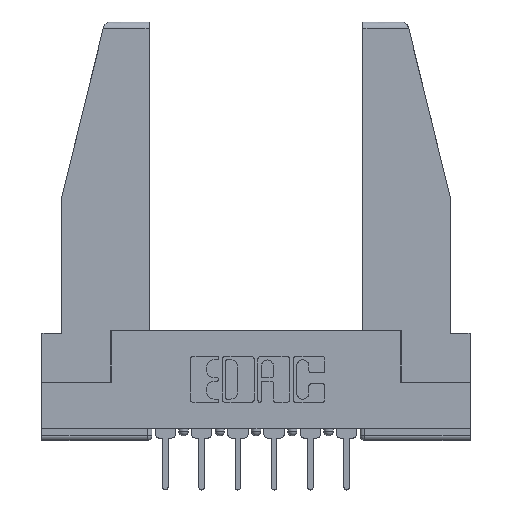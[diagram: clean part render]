
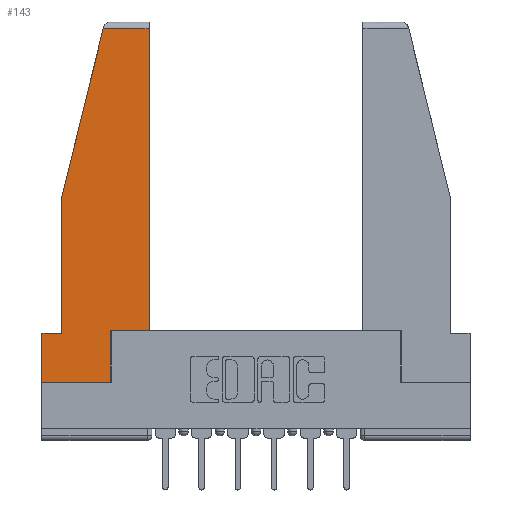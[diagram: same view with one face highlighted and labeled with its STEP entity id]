
A CAD part, top view. The second image highlights one B-rep face of the part: STEP entity #143.
In plain terms, the highlighted planar face has unit normal (0, 0, 1).
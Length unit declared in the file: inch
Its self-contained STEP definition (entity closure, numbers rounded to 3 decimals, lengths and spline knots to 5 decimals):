
#40 = CARTESIAN_POINT ( 'NONE',  ( 0.086, 0.8, 0. ) ) ;
#143 = ADVANCED_FACE ( 'NONE', ( #2385 ), #4320, .T. ) ;
#288 = VECTOR ( 'NONE', #3792, 39.37008 ) ;
#303 = CARTESIAN_POINT ( 'NONE',  ( 0.461, 0.223, 0. ) ) ;
#345 = CARTESIAN_POINT ( 'NONE',  ( 0.461, 1.52, 0. ) ) ;
#422 = VECTOR ( 'NONE', #2102, 39.37008 ) ;
#508 = AXIS2_PLACEMENT_3D ( 'NONE', #5173, #573, #6097 ) ;
#573 = DIRECTION ( 'NONE',  ( 0., 0., 1. ) ) ;
#831 = DIRECTION ( 'NONE',  ( -1., 0., 0. ) ) ;
#861 = ORIENTED_EDGE ( 'NONE', *, *, #2878, .T. ) ;
#1051 = VERTEX_POINT ( 'NONE', #1558 ) ;
#1068 = VECTOR ( 'NONE', #8438, 39.37008 ) ;
#1253 = EDGE_CURVE ( 'NONE', #8817, #5682, #1731, .T. ) ;
#1558 = CARTESIAN_POINT ( 'NONE',  ( 0., 0.21, 0. ) ) ;
#1731 = LINE ( 'NONE', #5439, #9088 ) ;
#1768 = ORIENTED_EDGE ( 'NONE', *, *, #2633, .T. ) ;
#1796 = LINE ( 'NONE', #7311, #1068 ) ;
#2012 = ORIENTED_EDGE ( 'NONE', *, *, #7397, .T. ) ;
#2063 = CARTESIAN_POINT ( 'NONE',  ( 0.461, 0.223, 0. ) ) ;
#2102 = DIRECTION ( 'NONE',  ( -1., 0., 0. ) ) ;
#2117 = CARTESIAN_POINT ( 'NONE',  ( 0.297, 0., 0. ) ) ;
#2385 = FACE_OUTER_BOUND ( 'NONE', #8413, .T. ) ;
#2633 = EDGE_CURVE ( 'NONE', #8666, #1051, #5809, .T. ) ;
#2878 = EDGE_CURVE ( 'NONE', #6167, #11511, #4934, .T. ) ;
#3441 = CARTESIAN_POINT ( 'NONE',  ( 0., 0., 0. ) ) ;
#3508 = CARTESIAN_POINT ( 'NONE',  ( 0.2636, 1.52, 0. ) ) ;
#3607 = EDGE_CURVE ( 'NONE', #11172, #5888, #1796, .T. ) ;
#3792 = DIRECTION ( 'NONE',  ( 0., 1., 0. ) ) ;
#4117 = VECTOR ( 'NONE', #8696, 39.37008 ) ;
#4271 = ORIENTED_EDGE ( 'NONE', *, *, #3607, .T. ) ;
#4320 = PLANE ( 'NONE',  #508 ) ;
#4495 = CARTESIAN_POINT ( 'NONE',  ( 0.086, 0.8, 0. ) ) ;
#4589 = CARTESIAN_POINT ( 'NONE',  ( 0.086, 0.21, 0. ) ) ;
#4756 = CARTESIAN_POINT ( 'NONE',  ( 0.297, 0.223, 0. ) ) ;
#4868 = EDGE_CURVE ( 'NONE', #5888, #6167, #8557, .T. ) ;
#4934 = LINE ( 'NONE', #4756, #6056 ) ;
#4969 = LINE ( 'NONE', #2063, #4117 ) ;
#5173 = CARTESIAN_POINT ( 'NONE',  ( 0., 0., 0. ) ) ;
#5438 = ORIENTED_EDGE ( 'NONE', *, *, #1253, .T. ) ;
#5439 = CARTESIAN_POINT ( 'NONE',  ( 0., 1.52, 0. ) ) ;
#5673 = LINE ( 'NONE', #8250, #9230 ) ;
#5674 = DIRECTION ( 'NONE',  ( 1., 0., 0. ) ) ;
#5682 = VERTEX_POINT ( 'NONE', #3508 ) ;
#5687 = DIRECTION ( 'NONE',  ( 0., -1., 0. ) ) ;
#5702 = VECTOR ( 'NONE', #5687, 39.37008 ) ;
#5769 = ORIENTED_EDGE ( 'NONE', *, *, #7533, .T. ) ;
#5804 = VERTEX_POINT ( 'NONE', #4495 ) ;
#5809 = LINE ( 'NONE', #7652, #422 ) ;
#5888 = VERTEX_POINT ( 'NONE', #2117 ) ;
#5933 = EDGE_CURVE ( 'NONE', #11511, #8817, #4969, .T. ) ;
#6056 = VECTOR ( 'NONE', #5674, 39.37008 ) ;
#6097 = DIRECTION ( 'NONE',  ( 1., 0., 0. ) ) ;
#6167 = VERTEX_POINT ( 'NONE', #7395 ) ;
#6293 = ORIENTED_EDGE ( 'NONE', *, *, #5933, .T. ) ;
#6838 = LINE ( 'NONE', #7761, #8831 ) ;
#7311 = CARTESIAN_POINT ( 'NONE',  ( 0., 0., 0. ) ) ;
#7395 = CARTESIAN_POINT ( 'NONE',  ( 0.297, 0.223, 0. ) ) ;
#7397 = EDGE_CURVE ( 'NONE', #5804, #8666, #11955, .T. ) ;
#7533 = EDGE_CURVE ( 'NONE', #1051, #11172, #6838, .T. ) ;
#7652 = CARTESIAN_POINT ( 'NONE',  ( 0., 0.21, 0. ) ) ;
#7761 = CARTESIAN_POINT ( 'NONE',  ( 0., 0.21, 0. ) ) ;
#7791 = EDGE_CURVE ( 'NONE', #5682, #5804, #5673, .T. ) ;
#8250 = CARTESIAN_POINT ( 'NONE',  ( 0.271, 1.55, 0. ) ) ;
#8371 = DIRECTION ( 'NONE',  ( -0.239, -0.971, 0. ) ) ;
#8413 = EDGE_LOOP ( 'NONE', ( #6293, #5438, #9698, #2012, #1768, #5769, #4271, #8726, #861 ) ) ;
#8438 = DIRECTION ( 'NONE',  ( 1., 0., 0. ) ) ;
#8557 = LINE ( 'NONE', #10256, #288 ) ;
#8666 = VERTEX_POINT ( 'NONE', #4589 ) ;
#8696 = DIRECTION ( 'NONE',  ( 0., 1., 0. ) ) ;
#8726 = ORIENTED_EDGE ( 'NONE', *, *, #4868, .T. ) ;
#8817 = VERTEX_POINT ( 'NONE', #345 ) ;
#8831 = VECTOR ( 'NONE', #11528, 39.37008 ) ;
#9088 = VECTOR ( 'NONE', #831, 39.37008 ) ;
#9230 = VECTOR ( 'NONE', #8371, 39.37008 ) ;
#9698 = ORIENTED_EDGE ( 'NONE', *, *, #7791, .T. ) ;
#10256 = CARTESIAN_POINT ( 'NONE',  ( 0.297, 0., 0. ) ) ;
#11172 = VERTEX_POINT ( 'NONE', #3441 ) ;
#11511 = VERTEX_POINT ( 'NONE', #303 ) ;
#11528 = DIRECTION ( 'NONE',  ( 0., -1., 0. ) ) ;
#11955 = LINE ( 'NONE', #40, #5702 ) ;
